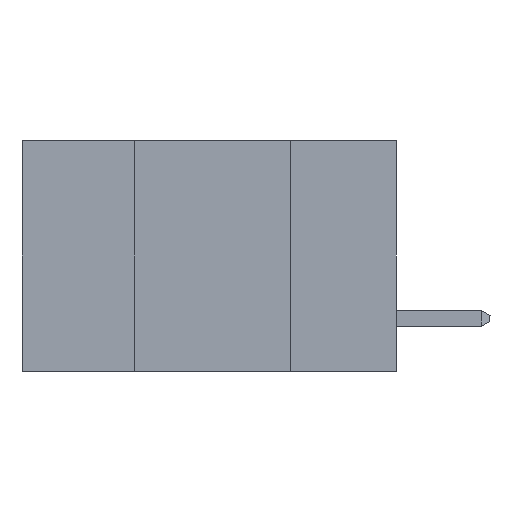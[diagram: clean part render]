
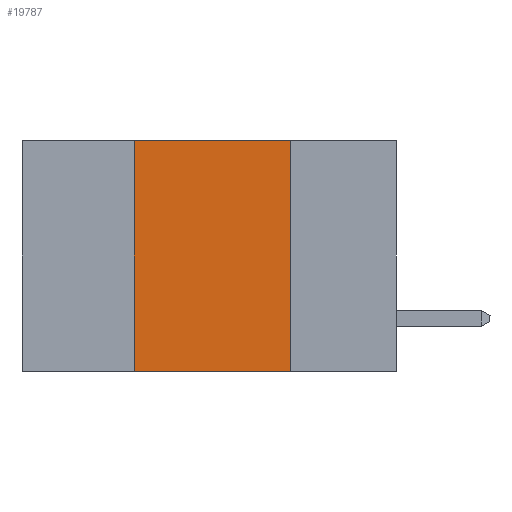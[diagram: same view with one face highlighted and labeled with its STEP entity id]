
A CAD part, left-side view. The second image highlights one B-rep face of the part: STEP entity #19787.
In plain terms, the highlighted planar face has unit normal (-1, 0, 0).
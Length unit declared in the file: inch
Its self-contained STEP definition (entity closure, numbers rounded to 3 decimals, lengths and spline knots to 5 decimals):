
#1007 = VECTOR ( 'NONE', #18510, 39.37008 ) ;
#1190 = VECTOR ( 'NONE', #2589, 39.37008 ) ;
#2285 = VERTEX_POINT ( 'NONE', #6970 ) ;
#2291 = ORIENTED_EDGE ( 'NONE', *, *, #11157, .F. ) ;
#2589 = DIRECTION ( 'NONE',  ( 0., -1., 0. ) ) ;
#3862 = VERTEX_POINT ( 'NONE', #23092 ) ;
#5141 = EDGE_CURVE ( 'NONE', #2285, #3862, #21299, .T. ) ;
#5217 = ORIENTED_EDGE ( 'NONE', *, *, #5141, .F. ) ;
#5636 = VECTOR ( 'NONE', #7981, 39.37008 ) ;
#5849 = CARTESIAN_POINT ( 'NONE',  ( 0., 0.42, -0.37 ) ) ;
#6970 = CARTESIAN_POINT ( 'NONE',  ( 0., 0.42, 0. ) ) ;
#7625 = CARTESIAN_POINT ( 'NONE',  ( 0., 0.42, -0.37 ) ) ;
#7957 = CARTESIAN_POINT ( 'NONE',  ( 0., 0.6, 0. ) ) ;
#7981 = DIRECTION ( 'NONE',  ( 0., 0., 1. ) ) ;
#9197 = LINE ( 'NONE', #18749, #1007 ) ;
#9857 = EDGE_CURVE ( 'NONE', #22948, #2285, #14944, .T. ) ;
#10075 = ORIENTED_EDGE ( 'NONE', *, *, #9857, .F. ) ;
#10198 = CARTESIAN_POINT ( 'NONE',  ( 0., 0.17, -0.37 ) ) ;
#10641 = FACE_OUTER_BOUND ( 'NONE', #21882, .T. ) ;
#10906 = VERTEX_POINT ( 'NONE', #10198 ) ;
#11157 = EDGE_CURVE ( 'NONE', #3862, #10906, #9197, .T. ) ;
#11237 = LINE ( 'NONE', #22258, #15405 ) ;
#11603 = EDGE_CURVE ( 'NONE', #22948, #10906, #11237, .T. ) ;
#12523 = AXIS2_PLACEMENT_3D ( 'NONE', #20204, #21659, #21785 ) ;
#12582 = PLANE ( 'NONE',  #12523 ) ;
#14944 = LINE ( 'NONE', #7625, #5636 ) ;
#15405 = VECTOR ( 'NONE', #24094, 39.37008 ) ;
#18510 = DIRECTION ( 'NONE',  ( 0., 0., -1. ) ) ;
#18749 = CARTESIAN_POINT ( 'NONE',  ( 0., 0.17, -0.37 ) ) ;
#19787 = ADVANCED_FACE ( 'NONE', ( #10641 ), #12582, .F. ) ;
#20204 = CARTESIAN_POINT ( 'NONE',  ( 0., 0.6, 0. ) ) ;
#21299 = LINE ( 'NONE', #7957, #1190 ) ;
#21659 = DIRECTION ( 'NONE',  ( 1., 0., 0. ) ) ;
#21785 = DIRECTION ( 'NONE',  ( 0., 0., -1. ) ) ;
#21882 = EDGE_LOOP ( 'NONE', ( #2291, #5217, #10075, #22335 ) ) ;
#22258 = CARTESIAN_POINT ( 'NONE',  ( 0., 0.6, -0.37 ) ) ;
#22335 = ORIENTED_EDGE ( 'NONE', *, *, #11603, .T. ) ;
#22948 = VERTEX_POINT ( 'NONE', #5849 ) ;
#23092 = CARTESIAN_POINT ( 'NONE',  ( 0., 0.17, 0. ) ) ;
#24094 = DIRECTION ( 'NONE',  ( 0., -1., 0. ) ) ;
